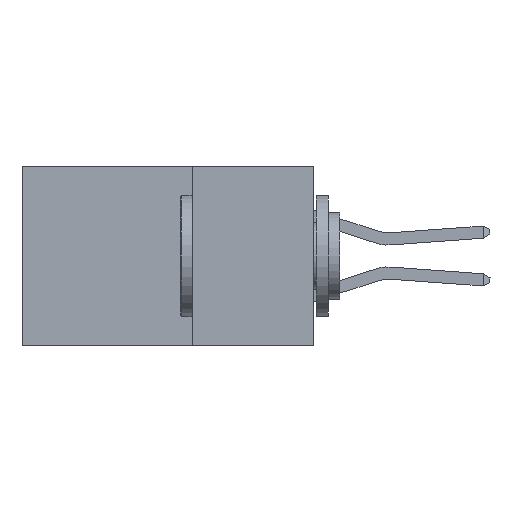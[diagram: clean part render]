
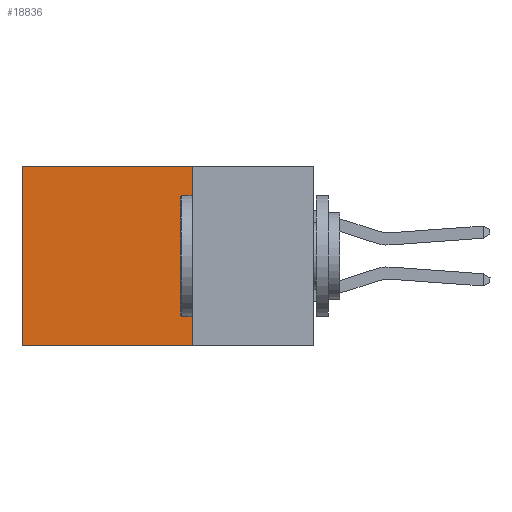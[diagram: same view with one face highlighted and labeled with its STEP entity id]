
A CAD part, left-side view. The second image highlights one B-rep face of the part: STEP entity #18836.
In plain terms, the highlighted planar face has unit normal (-1, 0, 0).
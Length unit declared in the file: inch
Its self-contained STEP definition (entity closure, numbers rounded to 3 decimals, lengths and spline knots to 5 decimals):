
#755 = CARTESIAN_POINT ( 'NONE',  ( 0.2875, 0.6, -0.37 ) ) ;
#1317 = CARTESIAN_POINT ( 'NONE',  ( 0.2875, 0.25, -0.37 ) ) ;
#1430 = DIRECTION ( 'NONE',  ( 0., 0., -1. ) ) ;
#1583 = EDGE_CURVE ( 'NONE', #14896, #10694, #18652, .T. ) ;
#2108 = LINE ( 'NONE', #9358, #13177 ) ;
#2160 = VECTOR ( 'NONE', #11073, 39.37008 ) ;
#4126 = ORIENTED_EDGE ( 'NONE', *, *, #8344, .T. ) ;
#5647 = DIRECTION ( 'NONE',  ( 0., 1., 0. ) ) ;
#7405 = EDGE_LOOP ( 'NONE', ( #20966, #20103, #7706, #4126 ) ) ;
#7706 = ORIENTED_EDGE ( 'NONE', *, *, #8158, .F. ) ;
#8158 = EDGE_CURVE ( 'NONE', #19969, #14896, #9808, .T. ) ;
#8344 = EDGE_CURVE ( 'NONE', #19969, #10390, #11452, .T. ) ;
#9171 = VECTOR ( 'NONE', #9181, 39.37008 ) ;
#9181 = DIRECTION ( 'NONE',  ( 0., 0., -1. ) ) ;
#9358 = CARTESIAN_POINT ( 'NONE',  ( 0.2875, 0.6, 0. ) ) ;
#9728 = PLANE ( 'NONE',  #15376 ) ;
#9808 = LINE ( 'NONE', #15342, #9171 ) ;
#10390 = VERTEX_POINT ( 'NONE', #12361 ) ;
#10694 = VERTEX_POINT ( 'NONE', #755 ) ;
#11073 = DIRECTION ( 'NONE',  ( 0., 1., 0. ) ) ;
#11257 = CARTESIAN_POINT ( 'NONE',  ( 0.2875, 0.25, -0.37 ) ) ;
#11452 = LINE ( 'NONE', #23992, #26330 ) ;
#12361 = CARTESIAN_POINT ( 'NONE',  ( 0.2875, 0.6, 0. ) ) ;
#13177 = VECTOR ( 'NONE', #23646, 39.37008 ) ;
#13915 = DIRECTION ( 'NONE',  ( 1., 0., 0. ) ) ;
#14896 = VERTEX_POINT ( 'NONE', #1317 ) ;
#15300 = CARTESIAN_POINT ( 'NONE',  ( 0.2875, 0.25, 0. ) ) ;
#15342 = CARTESIAN_POINT ( 'NONE',  ( 0.2875, 0.25, 0. ) ) ;
#15376 = AXIS2_PLACEMENT_3D ( 'NONE', #25996, #13915, #1430 ) ;
#18652 = LINE ( 'NONE', #11257, #2160 ) ;
#18836 = ADVANCED_FACE ( 'NONE', ( #25753 ), #9728, .F. ) ;
#19969 = VERTEX_POINT ( 'NONE', #15300 ) ;
#20103 = ORIENTED_EDGE ( 'NONE', *, *, #1583, .F. ) ;
#20966 = ORIENTED_EDGE ( 'NONE', *, *, #23769, .T. ) ;
#23646 = DIRECTION ( 'NONE',  ( 0., 0., -1. ) ) ;
#23769 = EDGE_CURVE ( 'NONE', #10390, #10694, #2108, .T. ) ;
#23992 = CARTESIAN_POINT ( 'NONE',  ( 0.2875, 0.25, 0. ) ) ;
#25753 = FACE_OUTER_BOUND ( 'NONE', #7405, .T. ) ;
#25996 = CARTESIAN_POINT ( 'NONE',  ( 0.2875, 0.25, 0. ) ) ;
#26330 = VECTOR ( 'NONE', #5647, 39.37008 ) ;
